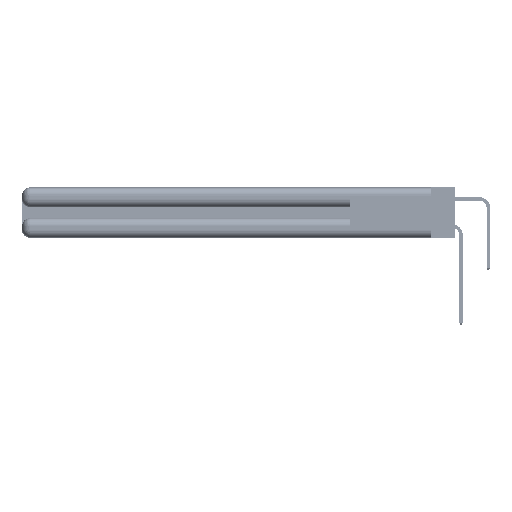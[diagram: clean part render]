
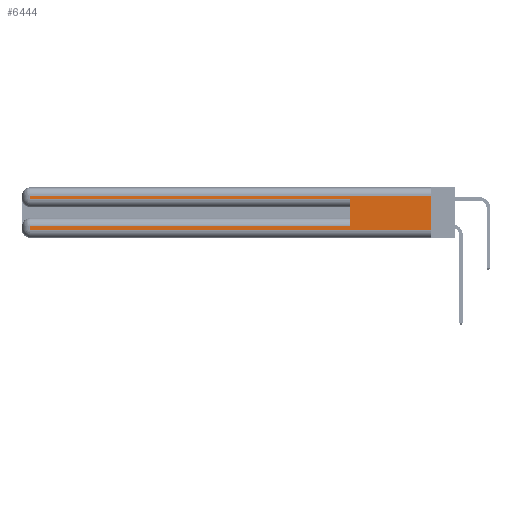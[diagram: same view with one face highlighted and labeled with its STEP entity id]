
A CAD part, left-side view. The second image highlights one B-rep face of the part: STEP entity #6444.
In plain terms, the highlighted planar face has unit normal (-1, 0, 0).
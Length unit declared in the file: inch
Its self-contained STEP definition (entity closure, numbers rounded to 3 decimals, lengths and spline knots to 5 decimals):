
#925 = LINE ( 'NONE', #17907, #33319 ) ;
#1041 = CARTESIAN_POINT ( 'NONE',  ( 0., 2.94, 0.285 ) ) ;
#1151 = DIRECTION ( 'NONE',  ( 0., 0., -1. ) ) ;
#1394 = VECTOR ( 'NONE', #46317, 39.37008 ) ;
#1857 = LINE ( 'NONE', #12476, #45568 ) ;
#2430 = VECTOR ( 'NONE', #45988, 39.37008 ) ;
#4030 = VERTEX_POINT ( 'NONE', #12106 ) ;
#4126 = ORIENTED_EDGE ( 'NONE', *, *, #49625, .T. ) ;
#4235 = ORIENTED_EDGE ( 'NONE', *, *, #44097, .F. ) ;
#5334 = LINE ( 'NONE', #38162, #1394 ) ;
#6088 = LINE ( 'NONE', #54473, #43907 ) ;
#6444 = ADVANCED_FACE ( 'NONE', ( #24655 ), #29778, .F. ) ;
#7805 = EDGE_CURVE ( 'NONE', #8519, #8840, #5334, .T. ) ;
#8519 = VERTEX_POINT ( 'NONE', #42717 ) ;
#8695 = VECTOR ( 'NONE', #26501, 39.37008 ) ;
#8840 = VERTEX_POINT ( 'NONE', #27434 ) ;
#8911 = CARTESIAN_POINT ( 'NONE',  ( 0., 2.94, 0.31 ) ) ;
#10363 = EDGE_CURVE ( 'NONE', #4030, #51984, #925, .T. ) ;
#12106 = CARTESIAN_POINT ( 'NONE',  ( 0., 0., 0.31 ) ) ;
#12476 = CARTESIAN_POINT ( 'NONE',  ( 0., 0., 0.085 ) ) ;
#13384 = EDGE_CURVE ( 'NONE', #28894, #8519, #1857, .T. ) ;
#16178 = DIRECTION ( 'NONE',  ( 0., 1., 0. ) ) ;
#16796 = EDGE_CURVE ( 'NONE', #8840, #51984, #54559, .T. ) ;
#17907 = CARTESIAN_POINT ( 'NONE',  ( 0., 0., 0.37 ) ) ;
#18363 = ORIENTED_EDGE ( 'NONE', *, *, #7805, .T. ) ;
#19559 = LINE ( 'NONE', #37375, #47513 ) ;
#19618 = AXIS2_PLACEMENT_3D ( 'NONE', #42426, #51196, #25690 ) ;
#19987 = EDGE_CURVE ( 'NONE', #29046, #40754, #44171, .T. ) ;
#21292 = CARTESIAN_POINT ( 'NONE',  ( 0., 0.6, 0.085 ) ) ;
#21809 = ORIENTED_EDGE ( 'NONE', *, *, #40083, .T. ) ;
#24655 = FACE_OUTER_BOUND ( 'NONE', #25418, .T. ) ;
#25138 = ORIENTED_EDGE ( 'NONE', *, *, #16796, .T. ) ;
#25266 = CARTESIAN_POINT ( 'NONE',  ( 0., 2.94, 0.37 ) ) ;
#25418 = EDGE_LOOP ( 'NONE', ( #53842, #21809, #4126, #41682, #4235, #42726, #18363, #25138 ) ) ;
#25690 = DIRECTION ( 'NONE',  ( 0., 0., -1. ) ) ;
#26501 = DIRECTION ( 'NONE',  ( 0., -1., 0. ) ) ;
#27434 = CARTESIAN_POINT ( 'NONE',  ( 0., 2.94, 0.06 ) ) ;
#28894 = VERTEX_POINT ( 'NONE', #21292 ) ;
#29046 = VERTEX_POINT ( 'NONE', #1041 ) ;
#29778 = PLANE ( 'NONE',  #19618 ) ;
#30250 = CARTESIAN_POINT ( 'NONE',  ( 0., 0., 0.06 ) ) ;
#32320 = VECTOR ( 'NONE', #38495, 39.37008 ) ;
#33319 = VECTOR ( 'NONE', #1151, 39.37008 ) ;
#33955 = DIRECTION ( 'NONE',  ( 0., 1., 0. ) ) ;
#34412 = CARTESIAN_POINT ( 'NONE',  ( 0., 0., 0.06 ) ) ;
#37375 = CARTESIAN_POINT ( 'NONE',  ( 0., 0.6, 0.145 ) ) ;
#38162 = CARTESIAN_POINT ( 'NONE',  ( 0., 2.94, 0.37 ) ) ;
#38301 = LINE ( 'NONE', #25266, #32320 ) ;
#38495 = DIRECTION ( 'NONE',  ( 0., 0., -1. ) ) ;
#40083 = EDGE_CURVE ( 'NONE', #4030, #54617, #6088, .T. ) ;
#40754 = VERTEX_POINT ( 'NONE', #43714 ) ;
#40975 = CARTESIAN_POINT ( 'NONE',  ( 0., 0., 0.285 ) ) ;
#41682 = ORIENTED_EDGE ( 'NONE', *, *, #19987, .T. ) ;
#42426 = CARTESIAN_POINT ( 'NONE',  ( 0., 0., 0.37 ) ) ;
#42717 = CARTESIAN_POINT ( 'NONE',  ( 0., 2.94, 0.085 ) ) ;
#42726 = ORIENTED_EDGE ( 'NONE', *, *, #13384, .T. ) ;
#43714 = CARTESIAN_POINT ( 'NONE',  ( 0., 0.6, 0.285 ) ) ;
#43907 = VECTOR ( 'NONE', #16178, 39.37008 ) ;
#44097 = EDGE_CURVE ( 'NONE', #28894, #40754, #19559, .T. ) ;
#44171 = LINE ( 'NONE', #40975, #2430 ) ;
#45568 = VECTOR ( 'NONE', #33955, 39.37008 ) ;
#45988 = DIRECTION ( 'NONE',  ( 0., -1., 0. ) ) ;
#46317 = DIRECTION ( 'NONE',  ( 0., 0., -1. ) ) ;
#47513 = VECTOR ( 'NONE', #50003, 39.37008 ) ;
#49625 = EDGE_CURVE ( 'NONE', #54617, #29046, #38301, .T. ) ;
#50003 = DIRECTION ( 'NONE',  ( 0., 0., 1. ) ) ;
#51196 = DIRECTION ( 'NONE',  ( 1., 0., 0. ) ) ;
#51984 = VERTEX_POINT ( 'NONE', #34412 ) ;
#53842 = ORIENTED_EDGE ( 'NONE', *, *, #10363, .F. ) ;
#54473 = CARTESIAN_POINT ( 'NONE',  ( 0., 0., 0.31 ) ) ;
#54559 = LINE ( 'NONE', #30250, #8695 ) ;
#54617 = VERTEX_POINT ( 'NONE', #8911 ) ;
